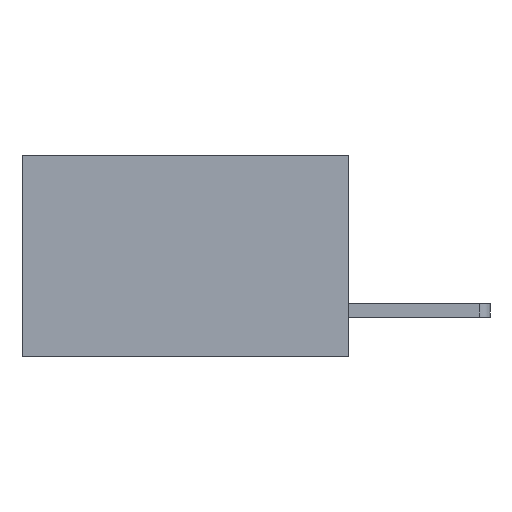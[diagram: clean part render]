
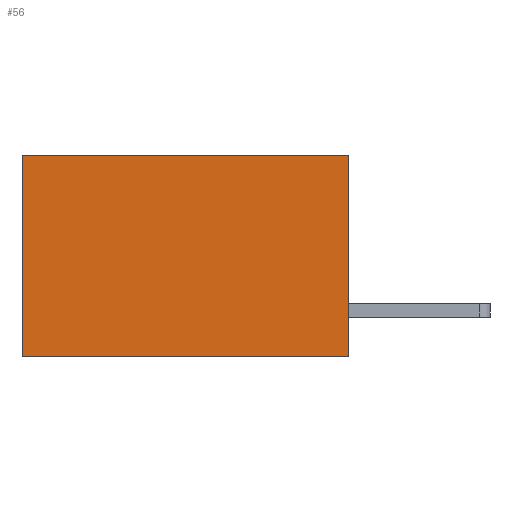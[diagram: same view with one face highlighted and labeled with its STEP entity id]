
A CAD part, left-side view. The second image highlights one B-rep face of the part: STEP entity #56.
In plain terms, the highlighted planar face has unit normal (-1, 0, 0).
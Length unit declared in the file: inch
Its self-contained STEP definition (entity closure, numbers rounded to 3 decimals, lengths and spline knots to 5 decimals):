
#56 = ADVANCED_FACE ( 'NONE', ( #7164 ), #5724, .F. ) ;
#572 = VERTEX_POINT ( 'NONE', #4488 ) ;
#614 = AXIS2_PLACEMENT_3D ( 'NONE', #5918, #1362, #5658 ) ;
#1362 = DIRECTION ( 'NONE',  ( 1., 0., 0. ) ) ;
#1673 = VECTOR ( 'NONE', #5521, 39.37008 ) ;
#2667 = ORIENTED_EDGE ( 'NONE', *, *, #3285, .F. ) ;
#2776 = LINE ( 'NONE', #5970, #6267 ) ;
#2852 = VERTEX_POINT ( 'NONE', #3707 ) ;
#2944 = ORIENTED_EDGE ( 'NONE', *, *, #4731, .F. ) ;
#3285 = EDGE_CURVE ( 'NONE', #572, #6820, #4858, .T. ) ;
#3707 = CARTESIAN_POINT ( 'NONE',  ( 0.2615, 0.6, 0. ) ) ;
#4077 = ORIENTED_EDGE ( 'NONE', *, *, #4319, .T. ) ;
#4254 = EDGE_CURVE ( 'NONE', #2852, #8197, #4742, .T. ) ;
#4300 = DIRECTION ( 'NONE',  ( 0., 0., -1. ) ) ;
#4319 = EDGE_CURVE ( 'NONE', #572, #2852, #5874, .T. ) ;
#4331 = VECTOR ( 'NONE', #7864, 39.37008 ) ;
#4488 = CARTESIAN_POINT ( 'NONE',  ( 0.2615, 0., 0. ) ) ;
#4645 = VECTOR ( 'NONE', #4300, 39.37008 ) ;
#4731 = EDGE_CURVE ( 'NONE', #6820, #8197, #2776, .T. ) ;
#4742 = LINE ( 'NONE', #6132, #1673 ) ;
#4774 = EDGE_LOOP ( 'NONE', ( #7372, #2944, #2667, #4077 ) ) ;
#4858 = LINE ( 'NONE', #5300, #4645 ) ;
#5175 = CARTESIAN_POINT ( 'NONE',  ( 0.2615, 0., -0.37 ) ) ;
#5300 = CARTESIAN_POINT ( 'NONE',  ( 0.2615, 0., -0.37 ) ) ;
#5521 = DIRECTION ( 'NONE',  ( 0., 0., -1. ) ) ;
#5658 = DIRECTION ( 'NONE',  ( 0., 0., -1. ) ) ;
#5724 = PLANE ( 'NONE',  #614 ) ;
#5874 = LINE ( 'NONE', #7868, #4331 ) ;
#5918 = CARTESIAN_POINT ( 'NONE',  ( 0.2615, 0., -0.37 ) ) ;
#5958 = DIRECTION ( 'NONE',  ( 0., 1., 0. ) ) ;
#5970 = CARTESIAN_POINT ( 'NONE',  ( 0.2615, 0., -0.37 ) ) ;
#6132 = CARTESIAN_POINT ( 'NONE',  ( 0.2615, 0.6, -0.37 ) ) ;
#6267 = VECTOR ( 'NONE', #5958, 39.37008 ) ;
#6820 = VERTEX_POINT ( 'NONE', #5175 ) ;
#7164 = FACE_OUTER_BOUND ( 'NONE', #4774, .T. ) ;
#7242 = CARTESIAN_POINT ( 'NONE',  ( 0.2615, 0.6, -0.37 ) ) ;
#7372 = ORIENTED_EDGE ( 'NONE', *, *, #4254, .T. ) ;
#7864 = DIRECTION ( 'NONE',  ( 0., 1., 0. ) ) ;
#7868 = CARTESIAN_POINT ( 'NONE',  ( 0.2615, 0., 0. ) ) ;
#8197 = VERTEX_POINT ( 'NONE', #7242 ) ;
